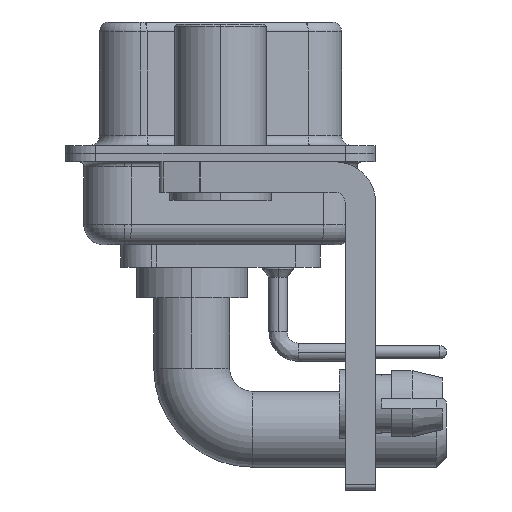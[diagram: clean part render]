
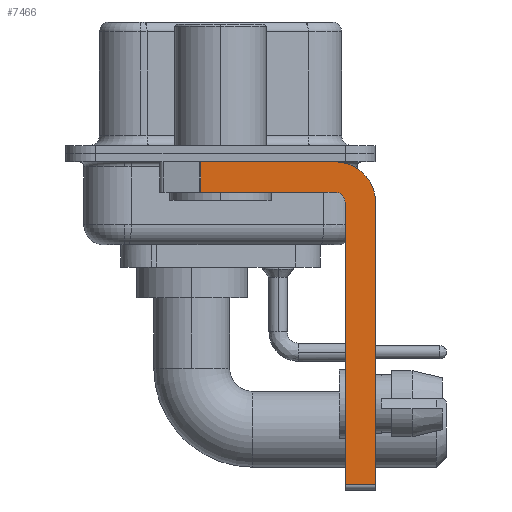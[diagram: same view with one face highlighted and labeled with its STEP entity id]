
A CAD part, left-side view. The second image highlights one B-rep face of the part: STEP entity #7466.
In plain terms, the highlighted planar face has unit normal (-1, 0, 0).
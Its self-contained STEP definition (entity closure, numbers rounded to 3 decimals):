
#1182 = VECTOR ( 'NONE', #13534, 1000. ) ;
#2174 = VERTEX_POINT ( 'NONE', #21480 ) ;
#2325 = CIRCLE ( 'NONE', #3647, 0.5 ) ;
#3647 = AXIS2_PLACEMENT_3D ( 'NONE', #7618, #11929, #7753 ) ;
#3891 = CARTESIAN_POINT ( 'NONE',  ( -2.9, -7.65, -2.4 ) ) ;
#4288 = CARTESIAN_POINT ( 'NONE',  ( -2.9, -5.65, -16.35 ) ) ;
#5728 = DIRECTION ( 'NONE',  ( 1., 0., 0. ) ) ;
#5779 = CARTESIAN_POINT ( 'NONE',  ( -2.9, -7.65, -2.4 ) ) ;
#5845 = VECTOR ( 'NONE', #14358, 1000. ) ;
#6409 = EDGE_CURVE ( 'NONE', #9465, #27293, #13432, .T. ) ;
#7466 = ADVANCED_FACE ( 'NONE', ( #26928 ), #20465, .F. ) ;
#7473 = ORIENTED_EDGE ( 'NONE', *, *, #16702, .F. ) ;
#7606 = AXIS2_PLACEMENT_3D ( 'NONE', #26795, #5728, #7807 ) ;
#7618 = CARTESIAN_POINT ( 'NONE',  ( -2.9, -5.65, -2.4 ) ) ;
#7694 = EDGE_CURVE ( 'NONE', #10449, #11412, #2325, .T. ) ;
#7753 = DIRECTION ( 'NONE',  ( 0., 0., 1. ) ) ;
#7807 = DIRECTION ( 'NONE',  ( 0., 0., -1. ) ) ;
#8030 = CARTESIAN_POINT ( 'NONE',  ( -2.9, 0.978, -1.9 ) ) ;
#8069 = EDGE_CURVE ( 'NONE', #9037, #8724, #22911, .T. ) ;
#8724 = VERTEX_POINT ( 'NONE', #23019 ) ;
#9037 = VERTEX_POINT ( 'NONE', #5779 ) ;
#9465 = VERTEX_POINT ( 'NONE', #20488 ) ;
#9739 = DIRECTION ( 'NONE',  ( 0., 0., -1. ) ) ;
#10202 = ORIENTED_EDGE ( 'NONE', *, *, #6409, .F. ) ;
#10449 = VERTEX_POINT ( 'NONE', #22587 ) ;
#10736 = VECTOR ( 'NONE', #10805, 1000. ) ;
#10805 = DIRECTION ( 'NONE',  ( 0., -1., 0. ) ) ;
#11412 = VERTEX_POINT ( 'NONE', #19186 ) ;
#11929 = DIRECTION ( 'NONE',  ( -1., 0., 0. ) ) ;
#11946 = VECTOR ( 'NONE', #21918, 1000. ) ;
#12364 = DIRECTION ( 'NONE',  ( 0., 0., -1. ) ) ;
#12454 = ORIENTED_EDGE ( 'NONE', *, *, #18684, .T. ) ;
#12858 = CARTESIAN_POINT ( 'NONE',  ( -2.9, -5.65, -0.4 ) ) ;
#13432 = LINE ( 'NONE', #26179, #11946 ) ;
#13534 = DIRECTION ( 'NONE',  ( 0., 1., 0. ) ) ;
#14175 = CARTESIAN_POINT ( 'NONE',  ( -2.9, -5.65, -2.4 ) ) ;
#14303 = CARTESIAN_POINT ( 'NONE',  ( -2.9, 0.978, -1.9 ) ) ;
#14335 = ORIENTED_EDGE ( 'NONE', *, *, #19995, .F. ) ;
#14358 = DIRECTION ( 'NONE',  ( 0., 0., 1. ) ) ;
#14745 = VECTOR ( 'NONE', #12364, 1000. ) ;
#15021 = ORIENTED_EDGE ( 'NONE', *, *, #23027, .F. ) ;
#16517 = DIRECTION ( 'NONE',  ( 0., 0., -1. ) ) ;
#16578 = CIRCLE ( 'NONE', #24530, 2. ) ;
#16702 = EDGE_CURVE ( 'NONE', #2174, #10449, #22961, .T. ) ;
#17258 = ORIENTED_EDGE ( 'NONE', *, *, #22051, .T. ) ;
#18607 = EDGE_LOOP ( 'NONE', ( #10202, #17258, #15021, #25120, #7473, #12454, #20277, #14335 ) ) ;
#18684 = EDGE_CURVE ( 'NONE', #2174, #8724, #21508, .T. ) ;
#19186 = CARTESIAN_POINT ( 'NONE',  ( -2.9, -5.65, -1.9 ) ) ;
#19684 = CARTESIAN_POINT ( 'NONE',  ( -2.9, -5.65, -1.9 ) ) ;
#19995 = EDGE_CURVE ( 'NONE', #27293, #9037, #16578, .T. ) ;
#20223 = VECTOR ( 'NONE', #16517, 1000. ) ;
#20277 = ORIENTED_EDGE ( 'NONE', *, *, #8069, .F. ) ;
#20465 = PLANE ( 'NONE',  #7606 ) ;
#20488 = CARTESIAN_POINT ( 'NONE',  ( -2.9, 0.978, -0.4 ) ) ;
#21480 = CARTESIAN_POINT ( 'NONE',  ( -2.9, -6.15, -16.35 ) ) ;
#21508 = LINE ( 'NONE', #4288, #10736 ) ;
#21918 = DIRECTION ( 'NONE',  ( 0., -1., 0. ) ) ;
#22051 = EDGE_CURVE ( 'NONE', #9465, #24115, #25362, .T. ) ;
#22587 = CARTESIAN_POINT ( 'NONE',  ( -2.9, -6.15, -2.4 ) ) ;
#22645 = DIRECTION ( 'NONE',  ( 1., 0., 0. ) ) ;
#22911 = LINE ( 'NONE', #3891, #14745 ) ;
#22961 = LINE ( 'NONE', #24887, #5845 ) ;
#23019 = CARTESIAN_POINT ( 'NONE',  ( -2.9, -7.65, -16.35 ) ) ;
#23027 = EDGE_CURVE ( 'NONE', #11412, #24115, #24219, .T. ) ;
#24115 = VERTEX_POINT ( 'NONE', #14303 ) ;
#24219 = LINE ( 'NONE', #19684, #1182 ) ;
#24530 = AXIS2_PLACEMENT_3D ( 'NONE', #14175, #22645, #9739 ) ;
#24887 = CARTESIAN_POINT ( 'NONE',  ( -2.9, -6.15, -16.6 ) ) ;
#25120 = ORIENTED_EDGE ( 'NONE', *, *, #7694, .F. ) ;
#25362 = LINE ( 'NONE', #8030, #20223 ) ;
#26179 = CARTESIAN_POINT ( 'NONE',  ( -2.9, 3., -0.4 ) ) ;
#26795 = CARTESIAN_POINT ( 'NONE',  ( -2.9, -5.65, -2.4 ) ) ;
#26928 = FACE_OUTER_BOUND ( 'NONE', #18607, .T. ) ;
#27293 = VERTEX_POINT ( 'NONE', #12858 ) ;
